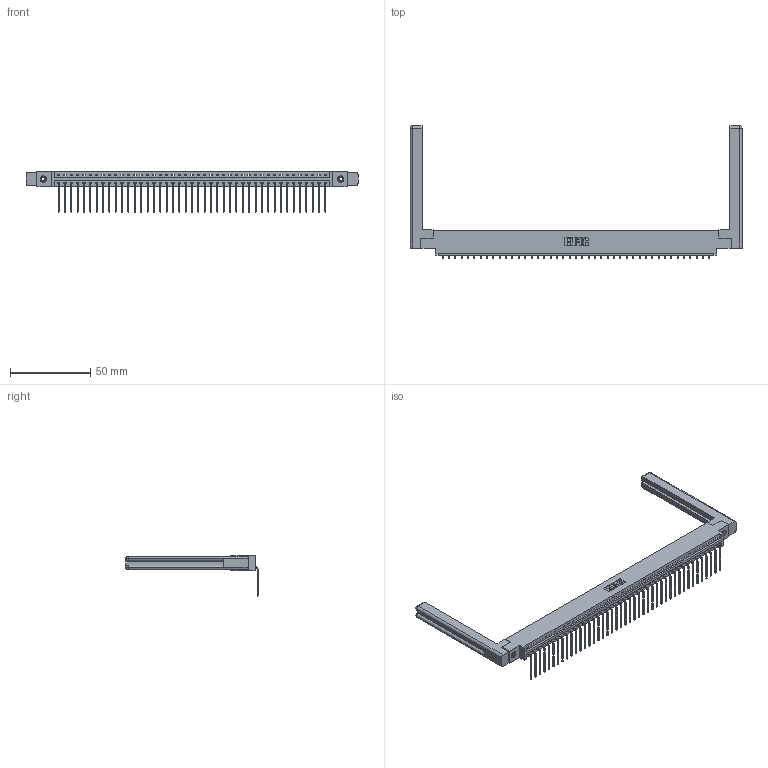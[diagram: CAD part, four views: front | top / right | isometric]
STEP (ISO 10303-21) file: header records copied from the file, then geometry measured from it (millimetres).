
FILE_DESCRIPTION (( 'STEP AP203' ), '1' );
FILE_NAME ('337-043-559-658.STEP', '2019-10-02T00:15:19', ( '' ), ( '' ), 'SwSTEP 2.0', 'SolidWorks 2016', '' );
FILE_SCHEMA (( 'CONFIG_CONTROL_DESIGN' ));
Length unit declared in the file: inch
Products named in the file (5): 337-043-559-658; 345-250-001_345-250-001-102; 337 Part_0.170 Offset - 0.156 Dia-TI; 345-292-001_558 559 Tail - 1; 307-220-058
Assembly tree (48 placements, depth 2):
  337-043-559-658
    337 Part_0.170 Offset - 0.156 Dia-TI
    345-292-001_558 559 Tail - 1  x43
    345-250-001_345-250-001-102  x2
    307-220-058  x2
Bounding box: 207.01 x 82.49 x 25.53 mm (x, y, z)
Volume: 28715.6 mm3; surface area: 28467.5 mm2
Topology: 48 solids, 48 shells, 3012 faces, 9019 edges, 5942 vertices
Faces by surface type: plane 2222, cylinder 766, cone 12, torus 12
Entity records: 34684 total; most frequent: CARTESIAN_POINT 6042, ORIENTED_EDGE 5960, DIRECTION 5102, EDGE_CURVE 2980, VECTOR 2804, LINE 2804, VERTEX_POINT 1978, AXIS2_PLACEMENT_3D 1149
